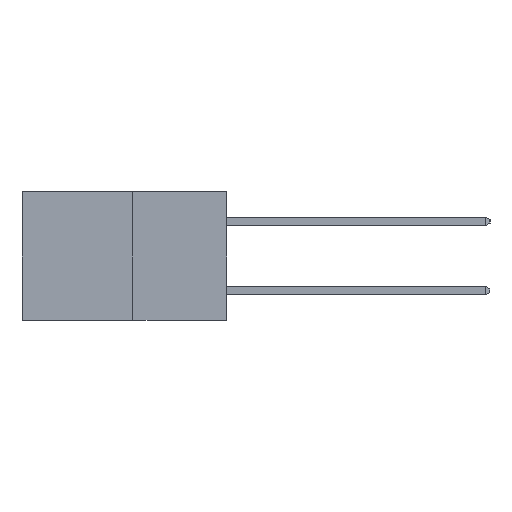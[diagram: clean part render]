
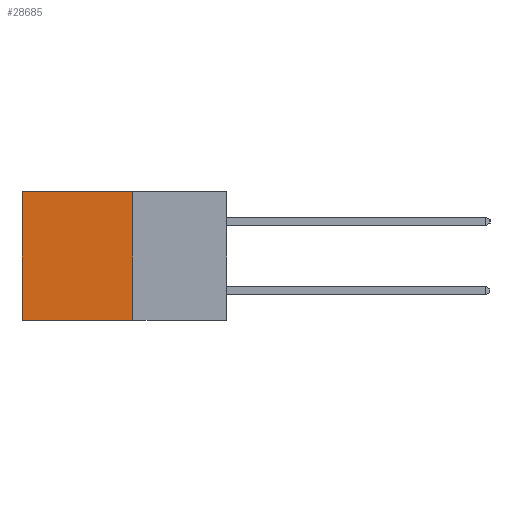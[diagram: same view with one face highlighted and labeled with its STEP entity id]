
A CAD part, left-side view. The second image highlights one B-rep face of the part: STEP entity #28685.
In plain terms, the highlighted planar face has unit normal (-1, 0, 0).
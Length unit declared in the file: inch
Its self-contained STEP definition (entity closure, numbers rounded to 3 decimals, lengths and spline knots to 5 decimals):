
#125 = VERTEX_POINT ( 'NONE', #10025 ) ;
#2171 = DIRECTION ( 'NONE',  ( 0., 0., -1. ) ) ;
#2699 = LINE ( 'NONE', #11842, #27638 ) ;
#2781 = CARTESIAN_POINT ( 'NONE',  ( 0.277, 0.59, -0.37 ) ) ;
#3033 = DIRECTION ( 'NONE',  ( 1., 0., 0. ) ) ;
#4606 = DIRECTION ( 'NONE',  ( 0., 0., -1. ) ) ;
#5675 = VECTOR ( 'NONE', #19153, 39.37008 ) ;
#6413 = LINE ( 'NONE', #23962, #5675 ) ;
#6449 = ORIENTED_EDGE ( 'NONE', *, *, #22509, .T. ) ;
#9509 = CARTESIAN_POINT ( 'NONE',  ( 0.277, 0.27, -0.37 ) ) ;
#9765 = EDGE_CURVE ( 'NONE', #125, #25917, #24549, .T. ) ;
#10025 = CARTESIAN_POINT ( 'NONE',  ( 0.277, 0.27, -0.37 ) ) ;
#11842 = CARTESIAN_POINT ( 'NONE',  ( 0.277, 0.59, -0.37 ) ) ;
#12050 = CARTESIAN_POINT ( 'NONE',  ( 0.277, 0.27, -0.37 ) ) ;
#12447 = ORIENTED_EDGE ( 'NONE', *, *, #30422, .F. ) ;
#12703 = LINE ( 'NONE', #9509, #24749 ) ;
#16082 = VERTEX_POINT ( 'NONE', #18469 ) ;
#17622 = CARTESIAN_POINT ( 'NONE',  ( 0.277, 0.27, -0.37 ) ) ;
#18469 = CARTESIAN_POINT ( 'NONE',  ( 0.277, 0.27, 0. ) ) ;
#19009 = FACE_OUTER_BOUND ( 'NONE', #26735, .T. ) ;
#19153 = DIRECTION ( 'NONE',  ( 0., 1., 0. ) ) ;
#20041 = DIRECTION ( 'NONE',  ( 0., 0., -1. ) ) ;
#20455 = AXIS2_PLACEMENT_3D ( 'NONE', #17622, #3033, #20041 ) ;
#22509 = EDGE_CURVE ( 'NONE', #27753, #25917, #2699, .T. ) ;
#23306 = EDGE_CURVE ( 'NONE', #16082, #27753, #6413, .T. ) ;
#23821 = VECTOR ( 'NONE', #24292, 39.37008 ) ;
#23962 = CARTESIAN_POINT ( 'NONE',  ( 0.277, 0.27, 0. ) ) ;
#24292 = DIRECTION ( 'NONE',  ( 0., 1., 0. ) ) ;
#24549 = LINE ( 'NONE', #12050, #23821 ) ;
#24717 = ORIENTED_EDGE ( 'NONE', *, *, #9765, .F. ) ;
#24749 = VECTOR ( 'NONE', #4606, 39.37008 ) ;
#25917 = VERTEX_POINT ( 'NONE', #2781 ) ;
#26735 = EDGE_LOOP ( 'NONE', ( #6449, #24717, #12447, #28042 ) ) ;
#27638 = VECTOR ( 'NONE', #2171, 39.37008 ) ;
#27753 = VERTEX_POINT ( 'NONE', #28619 ) ;
#28042 = ORIENTED_EDGE ( 'NONE', *, *, #23306, .T. ) ;
#28619 = CARTESIAN_POINT ( 'NONE',  ( 0.277, 0.59, 0. ) ) ;
#28685 = ADVANCED_FACE ( 'NONE', ( #19009 ), #29511, .F. ) ;
#29511 = PLANE ( 'NONE',  #20455 ) ;
#30422 = EDGE_CURVE ( 'NONE', #16082, #125, #12703, .T. ) ;
